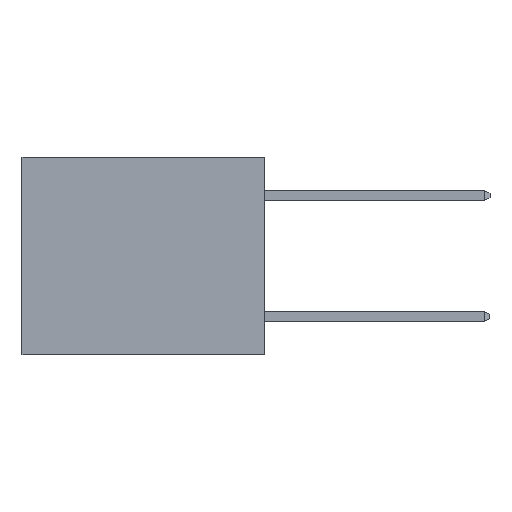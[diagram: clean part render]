
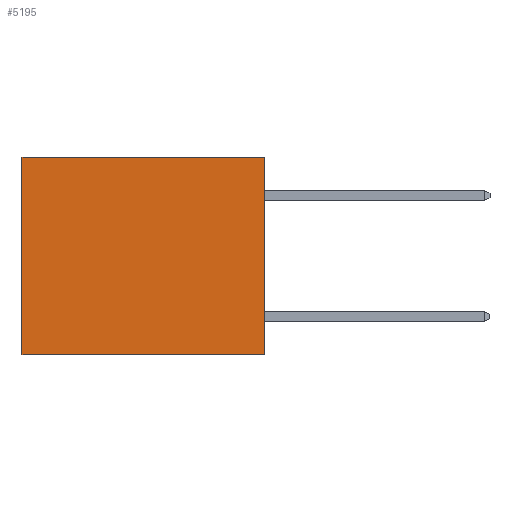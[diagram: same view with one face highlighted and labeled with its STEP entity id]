
A CAD part, left-side view. The second image highlights one B-rep face of the part: STEP entity #5195.
In plain terms, the highlighted planar face has unit normal (-1, 0, 0).
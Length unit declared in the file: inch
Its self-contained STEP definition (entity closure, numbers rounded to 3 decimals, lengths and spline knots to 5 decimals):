
#88 = VECTOR ( 'NONE', #12257, 39.37008 ) ;
#585 = DIRECTION ( 'NONE',  ( 0., 1., 0. ) ) ;
#916 = ORIENTED_EDGE ( 'NONE', *, *, #5662, .F. ) ;
#1039 = LINE ( 'NONE', #5963, #88 ) ;
#1749 = ORIENTED_EDGE ( 'NONE', *, *, #10080, .T. ) ;
#1931 = DIRECTION ( 'NONE',  ( 0., 0., -1. ) ) ;
#2427 = LINE ( 'NONE', #5797, #10731 ) ;
#3898 = EDGE_CURVE ( 'NONE', #11235, #6120, #4993, .T. ) ;
#4308 = FACE_OUTER_BOUND ( 'NONE', #12701, .T. ) ;
#4438 = CARTESIAN_POINT ( 'NONE',  ( 0.3165, 0., -0.49 ) ) ;
#4961 = CARTESIAN_POINT ( 'NONE',  ( 0.3165, 0., -0.49 ) ) ;
#4993 = LINE ( 'NONE', #7407, #9732 ) ;
#5071 = AXIS2_PLACEMENT_3D ( 'NONE', #4438, #11713, #5469 ) ;
#5195 = ADVANCED_FACE ( 'NONE', ( #4308 ), #10819, .F. ) ;
#5469 = DIRECTION ( 'NONE',  ( 0., 0., -1. ) ) ;
#5624 = EDGE_CURVE ( 'NONE', #5674, #13125, #11950, .T. ) ;
#5662 = EDGE_CURVE ( 'NONE', #13125, #6120, #1039, .T. ) ;
#5674 = VERTEX_POINT ( 'NONE', #12555 ) ;
#5797 = CARTESIAN_POINT ( 'NONE',  ( 0.3165, 0., 0. ) ) ;
#5963 = CARTESIAN_POINT ( 'NONE',  ( 0.3165, 0., -0.49 ) ) ;
#6120 = VERTEX_POINT ( 'NONE', #12324 ) ;
#6686 = CARTESIAN_POINT ( 'NONE',  ( 0.3165, 0., -0.49 ) ) ;
#7407 = CARTESIAN_POINT ( 'NONE',  ( 0.3165, 0.6, -0.49 ) ) ;
#9148 = VECTOR ( 'NONE', #1931, 39.37008 ) ;
#9349 = ORIENTED_EDGE ( 'NONE', *, *, #5624, .F. ) ;
#9732 = VECTOR ( 'NONE', #11555, 39.37008 ) ;
#10080 = EDGE_CURVE ( 'NONE', #5674, #11235, #2427, .T. ) ;
#10731 = VECTOR ( 'NONE', #585, 39.37008 ) ;
#10819 = PLANE ( 'NONE',  #5071 ) ;
#11235 = VERTEX_POINT ( 'NONE', #12400 ) ;
#11555 = DIRECTION ( 'NONE',  ( 0., 0., -1. ) ) ;
#11713 = DIRECTION ( 'NONE',  ( 1., 0., 0. ) ) ;
#11950 = LINE ( 'NONE', #4961, #9148 ) ;
#12257 = DIRECTION ( 'NONE',  ( 0., 1., 0. ) ) ;
#12324 = CARTESIAN_POINT ( 'NONE',  ( 0.3165, 0.6, -0.49 ) ) ;
#12400 = CARTESIAN_POINT ( 'NONE',  ( 0.3165, 0.6, 0. ) ) ;
#12555 = CARTESIAN_POINT ( 'NONE',  ( 0.3165, 0., 0. ) ) ;
#12701 = EDGE_LOOP ( 'NONE', ( #12936, #916, #9349, #1749 ) ) ;
#12936 = ORIENTED_EDGE ( 'NONE', *, *, #3898, .T. ) ;
#13125 = VERTEX_POINT ( 'NONE', #6686 ) ;
